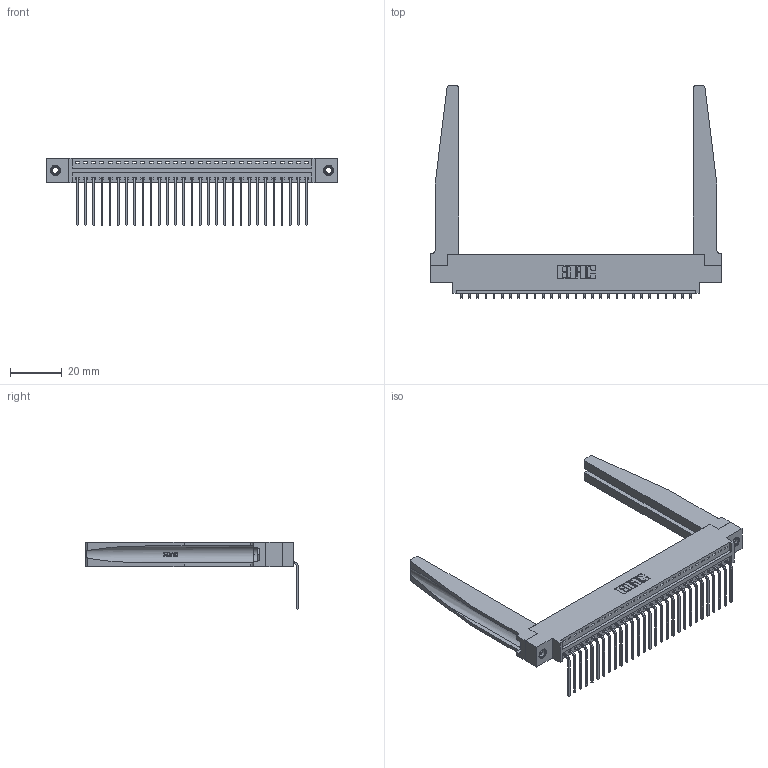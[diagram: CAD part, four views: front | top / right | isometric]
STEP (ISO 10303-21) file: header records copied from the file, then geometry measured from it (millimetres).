
FILE_DESCRIPTION (( 'STEP AP203' ), '1' );
FILE_NAME ('396-029-559-678.STEP', '2019-10-31T21:46:42', ( '' ), ( '' ), 'SwSTEP 2.0', 'SolidWorks 2016', '' );
FILE_SCHEMA (( 'CONFIG_CONTROL_DESIGN' ));
Length unit declared in the file: inch
Products named in the file (5): 346 Part_0.170 Offset - 0.156 Dia-TH; 345-292-001_558 559 Tail - 1; 346-220-078_345-220-078; 345-250-001_345-250-001-102; 396-029-559-678
Assembly tree (34 placements, depth 2):
  396-029-559-678
    346 Part_0.170 Offset - 0.156 Dia-TH
    345-292-001_558 559 Tail - 1  x29
    346-220-078_345-220-078  x2
    345-250-001_345-250-001-102  x2
Bounding box: 112.65 x 82.36 x 26.16 mm (x, y, z)
Volume: 17544.3 mm3; surface area: 20429.5 mm2
Topology: 34 solids, 34 shells, 2100 faces, 6227 edges, 4102 vertices
Faces by surface type: plane 1440, cylinder 608, bspline 36, cone 12, torus 4
Entity records: 24712 total; most frequent: CARTESIAN_POINT 5154, ORIENTED_EDGE 4006, DIRECTION 3547, EDGE_CURVE 2003, LINE 1661, VECTOR 1661, VERTEX_POINT 1328, AXIS2_PLACEMENT_3D 943
